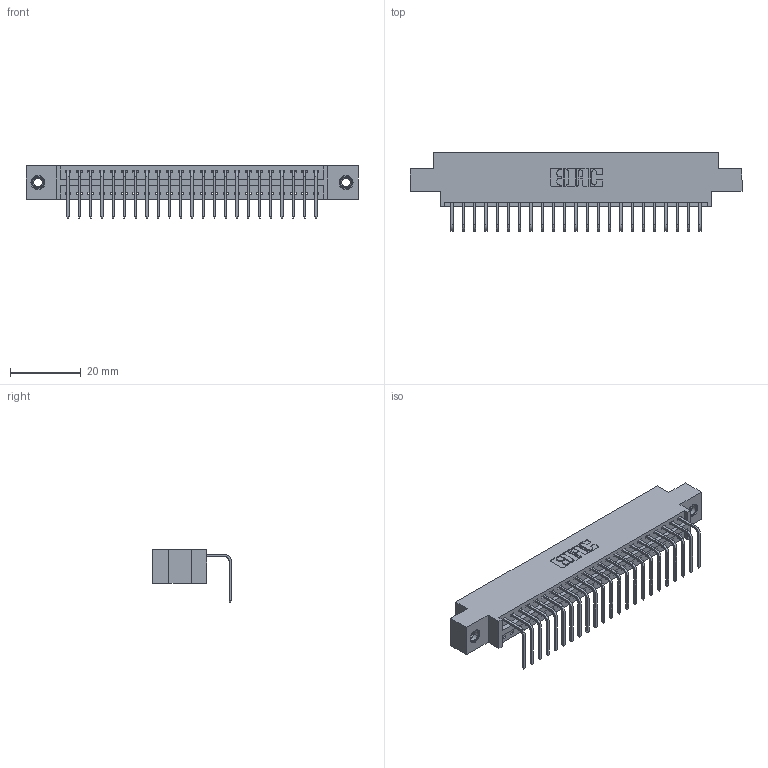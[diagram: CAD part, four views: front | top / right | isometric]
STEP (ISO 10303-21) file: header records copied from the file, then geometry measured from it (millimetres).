
FILE_DESCRIPTION (( 'STEP AP203' ), '1' );
FILE_NAME ('346-023-558-607.STEP', '2022-05-05T21:50:00', ( '' ), ( '' ), 'SwSTEP 2.0', 'SolidWorks 2020', '' );
FILE_SCHEMA (( 'CONFIG_CONTROL_DESIGN' ));
Length unit declared in the file: inch
Products named in the file (4): 346 Part_0.170 Offset - 0.156 Dia-TI; 346-023-558-607; 345-250-001_345-250-005-103; 345-292-001_558 Tail - 2
Assembly tree (26 placements, depth 2):
  346-023-558-607
    346 Part_0.170 Offset - 0.156 Dia-TI
    345-292-001_558 Tail - 2  x23
    345-250-001_345-250-005-103  x2
Bounding box: 93.6 x 22.16 x 14.73 mm (x, y, z)
Volume: 8737.1 mm3; surface area: 11367.4 mm2
Topology: 26 solids, 26 shells, 1566 faces, 4663 edges, 3070 vertices
Faces by surface type: plane 1078, cylinder 472, cone 12, torus 4
Entity records: 18234 total; most frequent: CARTESIAN_POINT 3116, ORIENTED_EDGE 3066, DIRECTION 2797, EDGE_CURVE 1533, VECTOR 1289, LINE 1289, VERTEX_POINT 1016, AXIS2_PLACEMENT_3D 754
